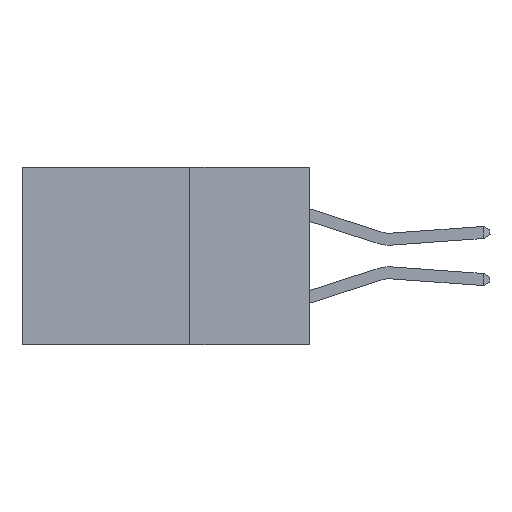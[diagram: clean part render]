
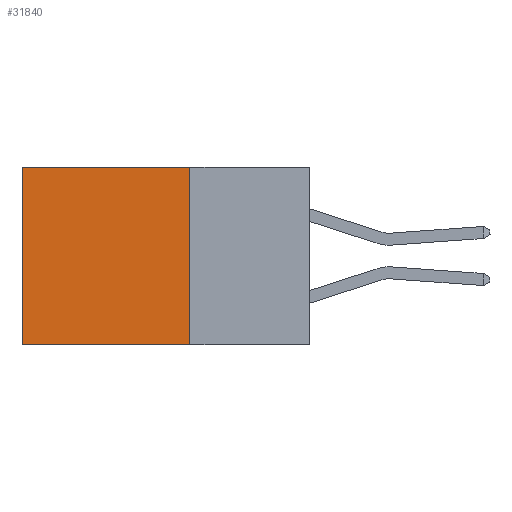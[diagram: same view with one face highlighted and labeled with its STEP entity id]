
A CAD part, left-side view. The second image highlights one B-rep face of the part: STEP entity #31840.
In plain terms, the highlighted planar face has unit normal (-1, 0, 0).
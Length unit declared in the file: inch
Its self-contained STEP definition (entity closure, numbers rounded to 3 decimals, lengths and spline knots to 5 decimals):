
#122 = PLANE ( 'NONE',  #28115 ) ;
#234 = CARTESIAN_POINT ( 'NONE',  ( 0.298, 0.25, 0. ) ) ;
#1042 = CARTESIAN_POINT ( 'NONE',  ( 0.298, 0.25, -0.37 ) ) ;
#2184 = VERTEX_POINT ( 'NONE', #26978 ) ;
#2474 = VECTOR ( 'NONE', #33657, 39.37008 ) ;
#2879 = DIRECTION ( 'NONE',  ( 0., 0., -1. ) ) ;
#3778 = VECTOR ( 'NONE', #24863, 39.37008 ) ;
#3938 = ORIENTED_EDGE ( 'NONE', *, *, #24590, .F. ) ;
#5394 = VERTEX_POINT ( 'NONE', #6576 ) ;
#6576 = CARTESIAN_POINT ( 'NONE',  ( 0.298, 0.6, -0.37 ) ) ;
#7647 = ORIENTED_EDGE ( 'NONE', *, *, #33058, .T. ) ;
#9216 = CARTESIAN_POINT ( 'NONE',  ( 0.298, 0.6, 0. ) ) ;
#11775 = CARTESIAN_POINT ( 'NONE',  ( 0.298, 0.25, 0. ) ) ;
#16115 = FACE_OUTER_BOUND ( 'NONE', #23573, .T. ) ;
#17358 = LINE ( 'NONE', #1042, #30462 ) ;
#17657 = LINE ( 'NONE', #11775, #3778 ) ;
#18553 = DIRECTION ( 'NONE',  ( 1., 0., 0. ) ) ;
#18743 = VECTOR ( 'NONE', #27466, 39.37008 ) ;
#19355 = DIRECTION ( 'NONE',  ( 0., 1., 0. ) ) ;
#20563 = CARTESIAN_POINT ( 'NONE',  ( 0.298, 0.25, 0. ) ) ;
#21676 = VERTEX_POINT ( 'NONE', #33581 ) ;
#23573 = EDGE_LOOP ( 'NONE', ( #30548, #30824, #3938, #7647 ) ) ;
#24145 = CARTESIAN_POINT ( 'NONE',  ( 0.298, 0.6, 0. ) ) ;
#24590 = EDGE_CURVE ( 'NONE', #2184, #21676, #30284, .T. ) ;
#24863 = DIRECTION ( 'NONE',  ( 0., 1., 0. ) ) ;
#26978 = CARTESIAN_POINT ( 'NONE',  ( 0.298, 0.25, 0. ) ) ;
#27466 = DIRECTION ( 'NONE',  ( 0., 0., -1. ) ) ;
#27502 = EDGE_CURVE ( 'NONE', #29818, #5394, #32601, .T. ) ;
#28115 = AXIS2_PLACEMENT_3D ( 'NONE', #234, #18553, #2879 ) ;
#29818 = VERTEX_POINT ( 'NONE', #24145 ) ;
#29919 = EDGE_CURVE ( 'NONE', #21676, #5394, #17358, .T. ) ;
#30284 = LINE ( 'NONE', #20563, #2474 ) ;
#30462 = VECTOR ( 'NONE', #19355, 39.37008 ) ;
#30548 = ORIENTED_EDGE ( 'NONE', *, *, #27502, .T. ) ;
#30824 = ORIENTED_EDGE ( 'NONE', *, *, #29919, .F. ) ;
#31840 = ADVANCED_FACE ( 'NONE', ( #16115 ), #122, .F. ) ;
#32601 = LINE ( 'NONE', #9216, #18743 ) ;
#33058 = EDGE_CURVE ( 'NONE', #2184, #29818, #17657, .T. ) ;
#33581 = CARTESIAN_POINT ( 'NONE',  ( 0.298, 0.25, -0.37 ) ) ;
#33657 = DIRECTION ( 'NONE',  ( 0., 0., -1. ) ) ;
